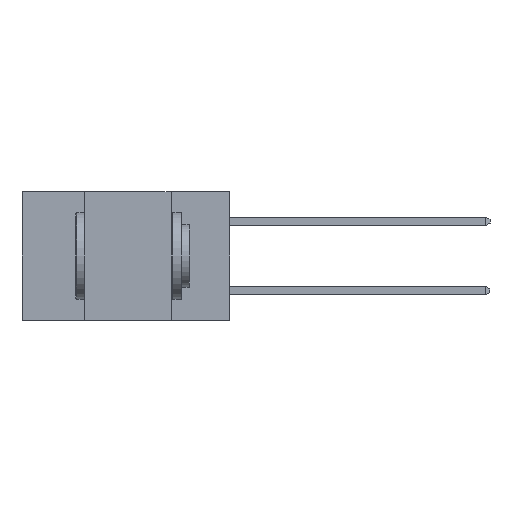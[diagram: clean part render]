
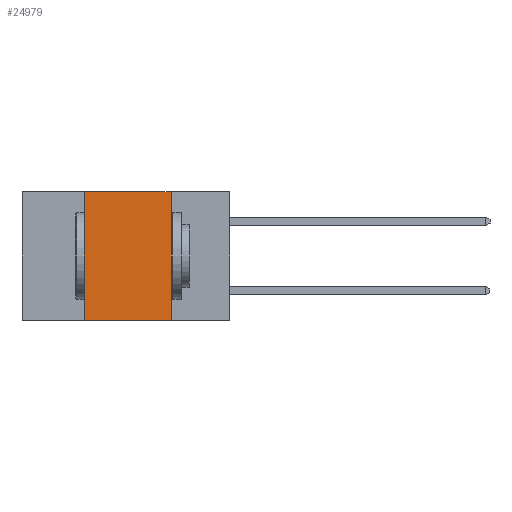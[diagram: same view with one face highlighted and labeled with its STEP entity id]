
A CAD part, left-side view. The second image highlights one B-rep face of the part: STEP entity #24979.
In plain terms, the highlighted planar face has unit normal (-1, 0, 0).
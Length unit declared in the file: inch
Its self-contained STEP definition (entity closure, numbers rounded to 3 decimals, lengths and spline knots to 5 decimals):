
#629 = CARTESIAN_POINT ( 'NONE',  ( 0., 0.17, 0. ) ) ;
#1227 = CARTESIAN_POINT ( 'NONE',  ( 0., 0.42, 0. ) ) ;
#4562 = EDGE_CURVE ( 'NONE', #23500, #20210, #21815, .T. ) ;
#5295 = AXIS2_PLACEMENT_3D ( 'NONE', #22964, #24857, #13532 ) ;
#5948 = LINE ( 'NONE', #22804, #15660 ) ;
#7027 = CARTESIAN_POINT ( 'NONE',  ( 0., 0.6, 0. ) ) ;
#7352 = ORIENTED_EDGE ( 'NONE', *, *, #7561, .F. ) ;
#7561 = EDGE_CURVE ( 'NONE', #10955, #7737, #20165, .T. ) ;
#7737 = VERTEX_POINT ( 'NONE', #24082 ) ;
#7816 = CARTESIAN_POINT ( 'NONE',  ( 0., 0.42, -0.37 ) ) ;
#8788 = EDGE_LOOP ( 'NONE', ( #7352, #13112, #24968, #10402 ) ) ;
#10402 = ORIENTED_EDGE ( 'NONE', *, *, #15456, .T. ) ;
#10955 = VERTEX_POINT ( 'NONE', #629 ) ;
#11429 = DIRECTION ( 'NONE',  ( 0., -1., 0. ) ) ;
#11719 = VECTOR ( 'NONE', #17272, 39.37008 ) ;
#12244 = CARTESIAN_POINT ( 'NONE',  ( 0., 0.17, 0. ) ) ;
#12794 = CARTESIAN_POINT ( 'NONE',  ( 0., 0.42, 0. ) ) ;
#13112 = ORIENTED_EDGE ( 'NONE', *, *, #14425, .F. ) ;
#13532 = DIRECTION ( 'NONE',  ( 0., 0., -1. ) ) ;
#14170 = DIRECTION ( 'NONE',  ( 0., 0., -1. ) ) ;
#14228 = VECTOR ( 'NONE', #16726, 39.37008 ) ;
#14425 = EDGE_CURVE ( 'NONE', #20210, #10955, #19269, .T. ) ;
#15147 = VECTOR ( 'NONE', #14170, 39.37008 ) ;
#15456 = EDGE_CURVE ( 'NONE', #23500, #7737, #5948, .T. ) ;
#15660 = VECTOR ( 'NONE', #11429, 39.37008 ) ;
#16726 = DIRECTION ( 'NONE',  ( 0., -1., 0. ) ) ;
#17272 = DIRECTION ( 'NONE',  ( 0., 0., 1. ) ) ;
#19269 = LINE ( 'NONE', #7027, #14228 ) ;
#20165 = LINE ( 'NONE', #12244, #15147 ) ;
#20210 = VERTEX_POINT ( 'NONE', #12794 ) ;
#21047 = PLANE ( 'NONE',  #5295 ) ;
#21815 = LINE ( 'NONE', #1227, #11719 ) ;
#22238 = FACE_OUTER_BOUND ( 'NONE', #8788, .T. ) ;
#22804 = CARTESIAN_POINT ( 'NONE',  ( 0., 0.6, -0.37 ) ) ;
#22964 = CARTESIAN_POINT ( 'NONE',  ( 0., 0.6, 0. ) ) ;
#23500 = VERTEX_POINT ( 'NONE', #7816 ) ;
#24082 = CARTESIAN_POINT ( 'NONE',  ( 0., 0.17, -0.37 ) ) ;
#24857 = DIRECTION ( 'NONE',  ( 1., 0., 0. ) ) ;
#24968 = ORIENTED_EDGE ( 'NONE', *, *, #4562, .F. ) ;
#24979 = ADVANCED_FACE ( 'NONE', ( #22238 ), #21047, .F. ) ;
